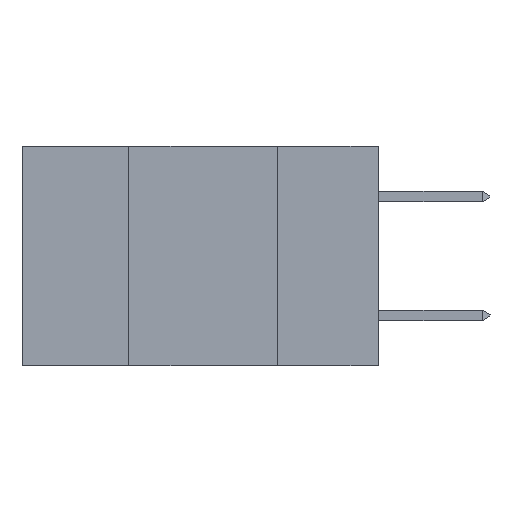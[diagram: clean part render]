
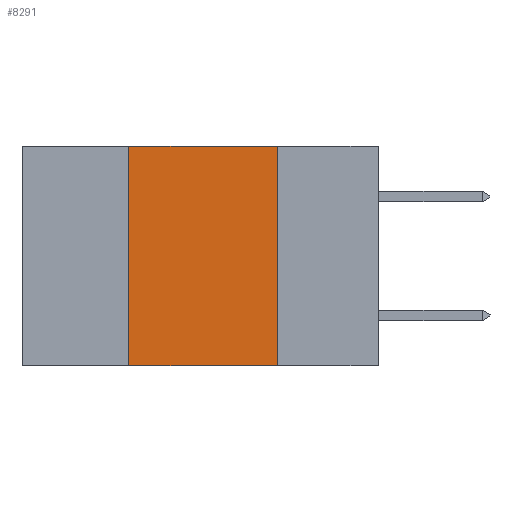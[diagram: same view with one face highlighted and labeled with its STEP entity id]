
A CAD part, left-side view. The second image highlights one B-rep face of the part: STEP entity #8291.
In plain terms, the highlighted planar face has unit normal (-1, 0, 0).
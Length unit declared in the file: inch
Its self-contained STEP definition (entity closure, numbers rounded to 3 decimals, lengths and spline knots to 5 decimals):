
#2433 = LINE ( 'NONE', #21821, #12996 ) ;
#3132 = CARTESIAN_POINT ( 'NONE',  ( 0., 0.6, -0.37 ) ) ;
#4079 = CARTESIAN_POINT ( 'NONE',  ( 0., 0.17, 0. ) ) ;
#7471 = LINE ( 'NONE', #18770, #27271 ) ;
#8291 = ADVANCED_FACE ( 'NONE', ( #28302 ), #9873, .F. ) ;
#8566 = EDGE_CURVE ( 'NONE', #29738, #20035, #20179, .T. ) ;
#9654 = CARTESIAN_POINT ( 'NONE',  ( 0., 0.6, 0. ) ) ;
#9873 = PLANE ( 'NONE',  #11351 ) ;
#10111 = EDGE_CURVE ( 'NONE', #19516, #20035, #2433, .T. ) ;
#11351 = AXIS2_PLACEMENT_3D ( 'NONE', #9654, #14520, #17122 ) ;
#11532 = DIRECTION ( 'NONE',  ( 0., 0., -1. ) ) ;
#11557 = DIRECTION ( 'NONE',  ( 0., -1., 0. ) ) ;
#11624 = EDGE_LOOP ( 'NONE', ( #15988, #11654, #31102, #13230 ) ) ;
#11654 = ORIENTED_EDGE ( 'NONE', *, *, #23508, .F. ) ;
#12797 = LINE ( 'NONE', #14264, #30144 ) ;
#12996 = VECTOR ( 'NONE', #11532, 39.37008 ) ;
#13230 = ORIENTED_EDGE ( 'NONE', *, *, #8566, .T. ) ;
#14264 = CARTESIAN_POINT ( 'NONE',  ( 0., 0.6, 0. ) ) ;
#14520 = DIRECTION ( 'NONE',  ( 1., 0., 0. ) ) ;
#15642 = EDGE_CURVE ( 'NONE', #29738, #32352, #7471, .T. ) ;
#15988 = ORIENTED_EDGE ( 'NONE', *, *, #10111, .F. ) ;
#17122 = DIRECTION ( 'NONE',  ( 0., 0., -1. ) ) ;
#17750 = CARTESIAN_POINT ( 'NONE',  ( 0., 0.42, 0. ) ) ;
#18561 = DIRECTION ( 'NONE',  ( 0., 0., 1. ) ) ;
#18770 = CARTESIAN_POINT ( 'NONE',  ( 0., 0.42, 0. ) ) ;
#19516 = VERTEX_POINT ( 'NONE', #4079 ) ;
#20035 = VERTEX_POINT ( 'NONE', #26987 ) ;
#20179 = LINE ( 'NONE', #3132, #28269 ) ;
#21821 = CARTESIAN_POINT ( 'NONE',  ( 0., 0.17, 0. ) ) ;
#23508 = EDGE_CURVE ( 'NONE', #32352, #19516, #12797, .T. ) ;
#24501 = DIRECTION ( 'NONE',  ( 0., -1., 0. ) ) ;
#26987 = CARTESIAN_POINT ( 'NONE',  ( 0., 0.17, -0.37 ) ) ;
#27271 = VECTOR ( 'NONE', #18561, 39.37008 ) ;
#28269 = VECTOR ( 'NONE', #24501, 39.37008 ) ;
#28302 = FACE_OUTER_BOUND ( 'NONE', #11624, .T. ) ;
#29738 = VERTEX_POINT ( 'NONE', #32472 ) ;
#30144 = VECTOR ( 'NONE', #11557, 39.37008 ) ;
#31102 = ORIENTED_EDGE ( 'NONE', *, *, #15642, .F. ) ;
#32352 = VERTEX_POINT ( 'NONE', #17750 ) ;
#32472 = CARTESIAN_POINT ( 'NONE',  ( 0., 0.42, -0.37 ) ) ;
